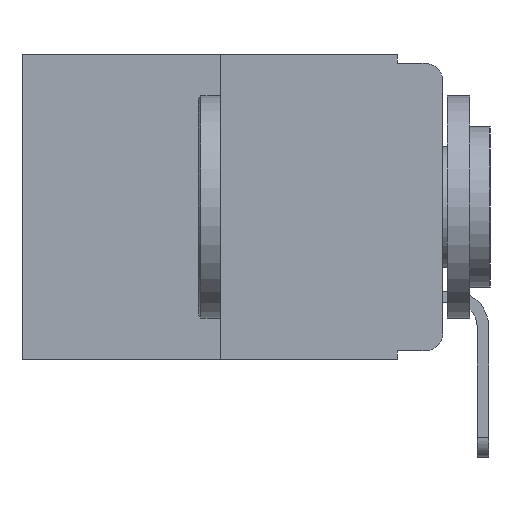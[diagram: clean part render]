
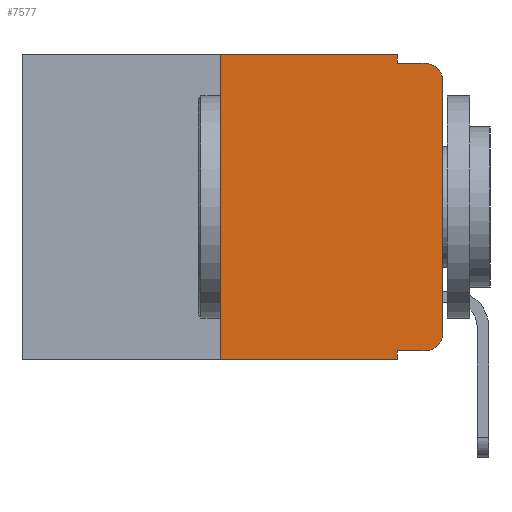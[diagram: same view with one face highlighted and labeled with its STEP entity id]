
A CAD part, left-side view. The second image highlights one B-rep face of the part: STEP entity #7577.
In plain terms, the highlighted planar face has unit normal (-1, 0, 0).
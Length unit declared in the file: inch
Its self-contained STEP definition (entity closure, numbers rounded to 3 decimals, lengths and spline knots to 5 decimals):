
#222 = CARTESIAN_POINT ( 'NONE',  ( 0., 0.02, -0.01 ) ) ;
#657 = CARTESIAN_POINT ( 'NONE',  ( 0., 0.051, 0. ) ) ;
#697 = VECTOR ( 'NONE', #16196, 39.37008 ) ;
#721 = EDGE_CURVE ( 'NONE', #972, #21895, #23160, .T. ) ;
#775 = VERTEX_POINT ( 'NONE', #25286 ) ;
#972 = VERTEX_POINT ( 'NONE', #17612 ) ;
#1590 = ORIENTED_EDGE ( 'NONE', *, *, #3864, .T. ) ;
#1661 = VECTOR ( 'NONE', #5654, 39.37008 ) ;
#1826 = LINE ( 'NONE', #7784, #11325 ) ;
#2218 = ORIENTED_EDGE ( 'NONE', *, *, #6669, .T. ) ;
#2493 = CARTESIAN_POINT ( 'NONE',  ( 0., 0.051, 0. ) ) ;
#2584 = CARTESIAN_POINT ( 'NONE',  ( 0., 0.02, -0.333 ) ) ;
#2605 = EDGE_CURVE ( 'NONE', #775, #21368, #18892, .T. ) ;
#2648 = EDGE_CURVE ( 'NONE', #9718, #2897, #8790, .T. ) ;
#2797 = EDGE_CURVE ( 'NONE', #21294, #21895, #1826, .T. ) ;
#2888 = AXIS2_PLACEMENT_3D ( 'NONE', #16806, #22943, #12844 ) ;
#2897 = VERTEX_POINT ( 'NONE', #9507 ) ;
#3371 = DIRECTION ( 'NONE',  ( 0., 0., 1. ) ) ;
#3726 = FACE_OUTER_BOUND ( 'NONE', #18650, .T. ) ;
#3864 = EDGE_CURVE ( 'NONE', #13510, #14366, #19391, .T. ) ;
#4090 = CARTESIAN_POINT ( 'NONE',  ( 0., 0.051, -0.01 ) ) ;
#5246 = DIRECTION ( 'NONE',  ( 0., 0., -1. ) ) ;
#5496 = LINE ( 'NONE', #13738, #25098 ) ;
#5654 = DIRECTION ( 'NONE',  ( 0., 0., -1. ) ) ;
#5777 = LINE ( 'NONE', #10093, #697 ) ;
#6312 = DIRECTION ( 'NONE',  ( 0., -1., 0. ) ) ;
#6669 = EDGE_CURVE ( 'NONE', #14729, #13510, #5777, .T. ) ;
#7577 = ADVANCED_FACE ( 'NONE', ( #3726 ), #16458, .F. ) ;
#7643 = DIRECTION ( 'NONE',  ( 0., 0., 1. ) ) ;
#7784 = CARTESIAN_POINT ( 'NONE',  ( 0., 0.051, -0.01 ) ) ;
#8790 = LINE ( 'NONE', #18339, #11964 ) ;
#8815 = DIRECTION ( 'NONE',  ( 0., 0., -1. ) ) ;
#8926 = AXIS2_PLACEMENT_3D ( 'NONE', #17336, #9221, #5246 ) ;
#9221 = DIRECTION ( 'NONE',  ( -1., 0., 0. ) ) ;
#9448 = VECTOR ( 'NONE', #8815, 39.37008 ) ;
#9507 = CARTESIAN_POINT ( 'NONE',  ( 0., 0.051, -0.343 ) ) ;
#9718 = VERTEX_POINT ( 'NONE', #22310 ) ;
#10093 = CARTESIAN_POINT ( 'NONE',  ( 0., 0.051, -0.333 ) ) ;
#11325 = VECTOR ( 'NONE', #22107, 39.37008 ) ;
#11556 = ORIENTED_EDGE ( 'NONE', *, *, #17514, .F. ) ;
#11964 = VECTOR ( 'NONE', #6312, 39.37008 ) ;
#12101 = CARTESIAN_POINT ( 'NONE',  ( 0., 0.051, -0.333 ) ) ;
#12172 = VECTOR ( 'NONE', #3371, 39.37008 ) ;
#12469 = EDGE_CURVE ( 'NONE', #14729, #2897, #18108, .T. ) ;
#12532 = ORIENTED_EDGE ( 'NONE', *, *, #22060, .F. ) ;
#12844 = DIRECTION ( 'NONE',  ( 0., 0., -1. ) ) ;
#13103 = DIRECTION ( 'NONE',  ( 0., 0., -1. ) ) ;
#13475 = ORIENTED_EDGE ( 'NONE', *, *, #24612, .T. ) ;
#13510 = VERTEX_POINT ( 'NONE', #2584 ) ;
#13738 = CARTESIAN_POINT ( 'NONE',  ( 0., 0.25, 0. ) ) ;
#13836 = CARTESIAN_POINT ( 'NONE',  ( 0., 0.473, 0. ) ) ;
#14366 = VERTEX_POINT ( 'NONE', #26082 ) ;
#14729 = VERTEX_POINT ( 'NONE', #12101 ) ;
#15170 = ORIENTED_EDGE ( 'NONE', *, *, #2605, .F. ) ;
#15354 = ORIENTED_EDGE ( 'NONE', *, *, #721, .T. ) ;
#16196 = DIRECTION ( 'NONE',  ( 0., -1., 0. ) ) ;
#16458 = PLANE ( 'NONE',  #23338 ) ;
#16806 = CARTESIAN_POINT ( 'NONE',  ( 0., 0.02, -0.313 ) ) ;
#17336 = CARTESIAN_POINT ( 'NONE',  ( 0., 0.02, -0.03 ) ) ;
#17514 = EDGE_CURVE ( 'NONE', #9718, #775, #5496, .T. ) ;
#17612 = CARTESIAN_POINT ( 'NONE',  ( 0., 0., -0.03 ) ) ;
#18108 = LINE ( 'NONE', #25270, #1661 ) ;
#18339 = CARTESIAN_POINT ( 'NONE',  ( 0., 0.473, -0.343 ) ) ;
#18650 = EDGE_LOOP ( 'NONE', ( #13475, #15354, #21685, #12532, #15170, #11556, #19141, #24089, #2218, #1590 ) ) ;
#18892 = LINE ( 'NONE', #13836, #23041 ) ;
#19141 = ORIENTED_EDGE ( 'NONE', *, *, #2648, .T. ) ;
#19238 = CARTESIAN_POINT ( 'NONE',  ( 0., 0., 0. ) ) ;
#19391 = CIRCLE ( 'NONE', #2888, 0.02 ) ;
#19536 = CARTESIAN_POINT ( 'NONE',  ( 0., 0.473, 0. ) ) ;
#21294 = VERTEX_POINT ( 'NONE', #4090 ) ;
#21368 = VERTEX_POINT ( 'NONE', #2493 ) ;
#21685 = ORIENTED_EDGE ( 'NONE', *, *, #2797, .F. ) ;
#21895 = VERTEX_POINT ( 'NONE', #222 ) ;
#22060 = EDGE_CURVE ( 'NONE', #21368, #21294, #22772, .T. ) ;
#22107 = DIRECTION ( 'NONE',  ( 0., -1., 0. ) ) ;
#22201 = DIRECTION ( 'NONE',  ( 1., 0., 0. ) ) ;
#22310 = CARTESIAN_POINT ( 'NONE',  ( 0., 0.25, -0.343 ) ) ;
#22772 = LINE ( 'NONE', #657, #9448 ) ;
#22943 = DIRECTION ( 'NONE',  ( -1., 0., 0. ) ) ;
#23041 = VECTOR ( 'NONE', #26081, 39.37008 ) ;
#23160 = CIRCLE ( 'NONE', #8926, 0.02 ) ;
#23338 = AXIS2_PLACEMENT_3D ( 'NONE', #19536, #22201, #13103 ) ;
#24089 = ORIENTED_EDGE ( 'NONE', *, *, #12469, .F. ) ;
#24612 = EDGE_CURVE ( 'NONE', #14366, #972, #24807, .T. ) ;
#24807 = LINE ( 'NONE', #19238, #12172 ) ;
#25098 = VECTOR ( 'NONE', #7643, 39.37008 ) ;
#25270 = CARTESIAN_POINT ( 'NONE',  ( 0., 0.051, 0. ) ) ;
#25286 = CARTESIAN_POINT ( 'NONE',  ( 0., 0.25, 0. ) ) ;
#26081 = DIRECTION ( 'NONE',  ( 0., -1., 0. ) ) ;
#26082 = CARTESIAN_POINT ( 'NONE',  ( 0., 0., -0.313 ) ) ;
